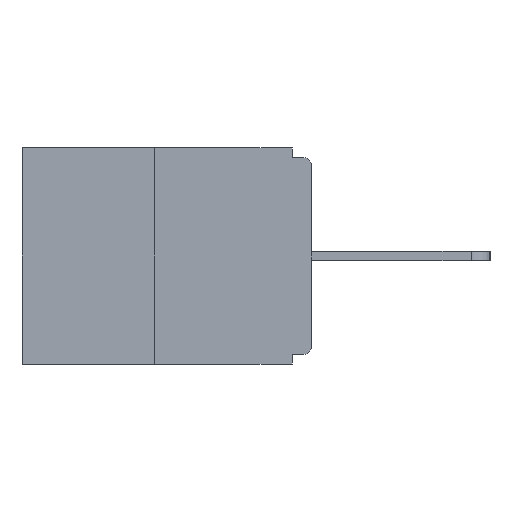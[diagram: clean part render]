
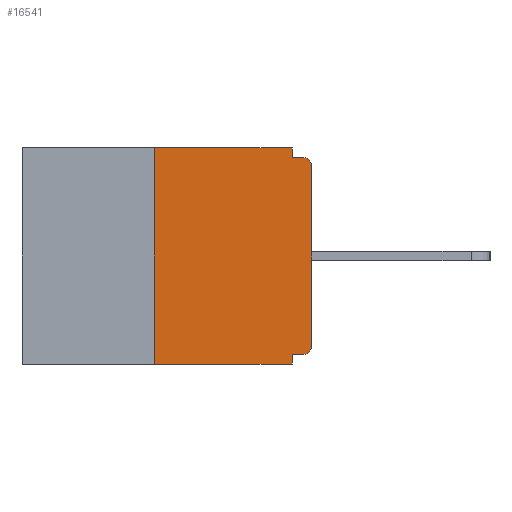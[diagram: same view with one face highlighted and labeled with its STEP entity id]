
A CAD part, left-side view. The second image highlights one B-rep face of the part: STEP entity #16541.
In plain terms, the highlighted planar face has unit normal (-1, 0, 0).
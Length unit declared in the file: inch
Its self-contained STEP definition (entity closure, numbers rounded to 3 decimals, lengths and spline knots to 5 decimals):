
#156 = CARTESIAN_POINT ( 'NONE',  ( 0., 0.46, 0. ) ) ;
#460 = DIRECTION ( 'NONE',  ( 0., 0., -1. ) ) ;
#584 = EDGE_CURVE ( 'NONE', #2983, #7637, #10238, .T. ) ;
#1562 = ORIENTED_EDGE ( 'NONE', *, *, #5846, .F. ) ;
#2037 = DIRECTION ( 'NONE',  ( -1., 0., 0. ) ) ;
#2483 = CIRCLE ( 'NONE', #16081, 0.015 ) ;
#2568 = VECTOR ( 'NONE', #16059, 39.37008 ) ;
#2606 = VECTOR ( 'NONE', #20454, 39.37008 ) ;
#2983 = VERTEX_POINT ( 'NONE', #12668 ) ;
#3027 = CARTESIAN_POINT ( 'NONE',  ( 0., 0.031, 0. ) ) ;
#3172 = CARTESIAN_POINT ( 'NONE',  ( 0., 0.46, 0. ) ) ;
#3280 = DIRECTION ( 'NONE',  ( 0., 0., 1. ) ) ;
#3286 = CARTESIAN_POINT ( 'NONE',  ( 0., 0., -0.328 ) ) ;
#3363 = ORIENTED_EDGE ( 'NONE', *, *, #14905, .T. ) ;
#3582 = VERTEX_POINT ( 'NONE', #16670 ) ;
#3813 = VECTOR ( 'NONE', #3280, 39.37008 ) ;
#4028 = LINE ( 'NONE', #20366, #6234 ) ;
#4063 = AXIS2_PLACEMENT_3D ( 'NONE', #15982, #10162, #15840 ) ;
#4349 = VECTOR ( 'NONE', #21987, 39.37008 ) ;
#4860 = CARTESIAN_POINT ( 'NONE',  ( 0., 0., 0. ) ) ;
#5326 = EDGE_CURVE ( 'NONE', #15735, #13419, #16867, .T. ) ;
#5398 = CARTESIAN_POINT ( 'NONE',  ( 0., 0.25, -0.343 ) ) ;
#5586 = LINE ( 'NONE', #3286, #2606 ) ;
#5846 = EDGE_CURVE ( 'NONE', #22535, #18931, #17112, .T. ) ;
#6137 = EDGE_CURVE ( 'NONE', #20432, #2983, #23926, .T. ) ;
#6234 = VECTOR ( 'NONE', #11566, 39.37008 ) ;
#6263 = EDGE_LOOP ( 'NONE', ( #17908, #22728, #3363, #1562, #23254, #23369, #17927, #11148, #12993, #12437 ) ) ;
#6562 = EDGE_CURVE ( 'NONE', #3582, #22535, #5586, .T. ) ;
#6687 = LINE ( 'NONE', #4860, #3813 ) ;
#7582 = VERTEX_POINT ( 'NONE', #21407 ) ;
#7637 = VERTEX_POINT ( 'NONE', #3027 ) ;
#7645 = EDGE_CURVE ( 'NONE', #7582, #15735, #6687, .T. ) ;
#7780 = VECTOR ( 'NONE', #16456, 39.37008 ) ;
#7813 = CARTESIAN_POINT ( 'NONE',  ( 0., 0., -0.03 ) ) ;
#8353 = CARTESIAN_POINT ( 'NONE',  ( 0., 0.031, -0.343 ) ) ;
#8916 = CARTESIAN_POINT ( 'NONE',  ( 0., 0.25, 0. ) ) ;
#9270 = DIRECTION ( 'NONE',  ( 1., 0., 0. ) ) ;
#9525 = DIRECTION ( 'NONE',  ( 0., 0., -1. ) ) ;
#10162 = DIRECTION ( 'NONE',  ( -1., 0., 0. ) ) ;
#10238 = LINE ( 'NONE', #3172, #2568 ) ;
#10869 = LINE ( 'NONE', #18289, #7780 ) ;
#10964 = VECTOR ( 'NONE', #13195, 39.37008 ) ;
#11049 = CARTESIAN_POINT ( 'NONE',  ( 0., 0.015, -0.313 ) ) ;
#11148 = ORIENTED_EDGE ( 'NONE', *, *, #5326, .T. ) ;
#11566 = DIRECTION ( 'NONE',  ( 0., -1., 0. ) ) ;
#11596 = CARTESIAN_POINT ( 'NONE',  ( 0., 0.031, -0.015 ) ) ;
#12437 = ORIENTED_EDGE ( 'NONE', *, *, #14358, .F. ) ;
#12498 = AXIS2_PLACEMENT_3D ( 'NONE', #156, #9270, #9525 ) ;
#12668 = CARTESIAN_POINT ( 'NONE',  ( 0., 0.25, 0. ) ) ;
#12993 = ORIENTED_EDGE ( 'NONE', *, *, #15963, .F. ) ;
#13195 = DIRECTION ( 'NONE',  ( 0., -1., 0. ) ) ;
#13419 = VERTEX_POINT ( 'NONE', #18454 ) ;
#14358 = EDGE_CURVE ( 'NONE', #7637, #14545, #10869, .T. ) ;
#14545 = VERTEX_POINT ( 'NONE', #11596 ) ;
#14905 = EDGE_CURVE ( 'NONE', #20432, #18931, #4028, .T. ) ;
#14990 = FACE_OUTER_BOUND ( 'NONE', #6263, .T. ) ;
#15391 = DIRECTION ( 'NONE',  ( 0., 0., -1. ) ) ;
#15735 = VERTEX_POINT ( 'NONE', #7813 ) ;
#15840 = DIRECTION ( 'NONE',  ( 0., 0., -1. ) ) ;
#15963 = EDGE_CURVE ( 'NONE', #14545, #13419, #18035, .T. ) ;
#15982 = CARTESIAN_POINT ( 'NONE',  ( 0., 0.015, -0.03 ) ) ;
#16059 = DIRECTION ( 'NONE',  ( 0., -1., 0. ) ) ;
#16081 = AXIS2_PLACEMENT_3D ( 'NONE', #11049, #2037, #460 ) ;
#16184 = CARTESIAN_POINT ( 'NONE',  ( 0., 0., -0.015 ) ) ;
#16456 = DIRECTION ( 'NONE',  ( 0., 0., -1. ) ) ;
#16541 = ADVANCED_FACE ( 'NONE', ( #14990 ), #20971, .F. ) ;
#16670 = CARTESIAN_POINT ( 'NONE',  ( 0., 0.015, -0.328 ) ) ;
#16867 = CIRCLE ( 'NONE', #4063, 0.015 ) ;
#17112 = LINE ( 'NONE', #8353, #21103 ) ;
#17908 = ORIENTED_EDGE ( 'NONE', *, *, #584, .F. ) ;
#17927 = ORIENTED_EDGE ( 'NONE', *, *, #7645, .T. ) ;
#18035 = LINE ( 'NONE', #16184, #10964 ) ;
#18250 = CARTESIAN_POINT ( 'NONE',  ( 0., 0.031, -0.343 ) ) ;
#18289 = CARTESIAN_POINT ( 'NONE',  ( 0., 0.031, 0. ) ) ;
#18454 = CARTESIAN_POINT ( 'NONE',  ( 0., 0.015, -0.015 ) ) ;
#18931 = VERTEX_POINT ( 'NONE', #18250 ) ;
#20366 = CARTESIAN_POINT ( 'NONE',  ( 0., 0.46, -0.343 ) ) ;
#20432 = VERTEX_POINT ( 'NONE', #5398 ) ;
#20454 = DIRECTION ( 'NONE',  ( 0., 1., 0. ) ) ;
#20971 = PLANE ( 'NONE',  #12498 ) ;
#21103 = VECTOR ( 'NONE', #15391, 39.37008 ) ;
#21327 = CARTESIAN_POINT ( 'NONE',  ( 0., 0.031, -0.328 ) ) ;
#21407 = CARTESIAN_POINT ( 'NONE',  ( 0., 0., -0.313 ) ) ;
#21671 = EDGE_CURVE ( 'NONE', #3582, #7582, #2483, .T. ) ;
#21987 = DIRECTION ( 'NONE',  ( 0., 0., 1. ) ) ;
#22535 = VERTEX_POINT ( 'NONE', #21327 ) ;
#22728 = ORIENTED_EDGE ( 'NONE', *, *, #6137, .F. ) ;
#23254 = ORIENTED_EDGE ( 'NONE', *, *, #6562, .F. ) ;
#23369 = ORIENTED_EDGE ( 'NONE', *, *, #21671, .T. ) ;
#23926 = LINE ( 'NONE', #8916, #4349 ) ;
